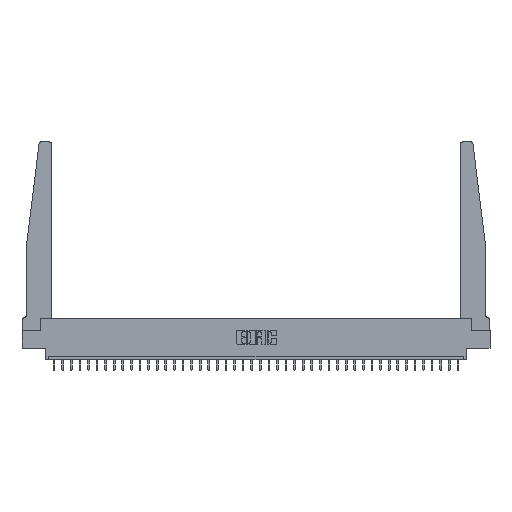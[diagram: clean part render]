
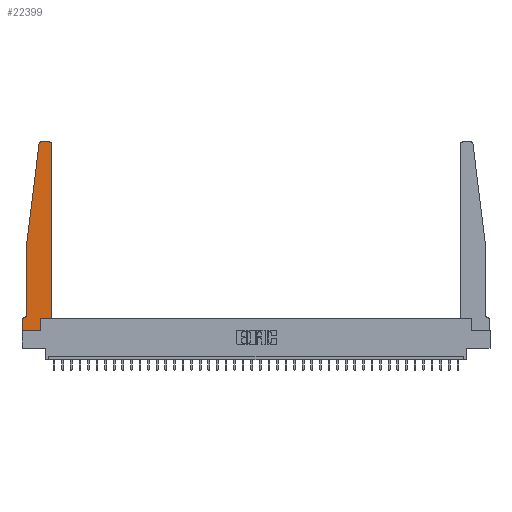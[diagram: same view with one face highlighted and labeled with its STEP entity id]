
A CAD part, top view. The second image highlights one B-rep face of the part: STEP entity #22399.
In plain terms, the highlighted planar face has unit normal (0, 0, 1).
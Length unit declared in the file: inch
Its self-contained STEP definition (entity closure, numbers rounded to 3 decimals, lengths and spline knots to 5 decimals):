
#115 = CARTESIAN_POINT ( 'NONE',  ( 0., 0.1875, 0.37 ) ) ;
#908 = EDGE_CURVE ( 'NONE', #25852, #27586, #5501, .T. ) ;
#1175 = ORIENTED_EDGE ( 'NONE', *, *, #10447, .T. ) ;
#1388 = CARTESIAN_POINT ( 'NONE',  ( 0.065, 0.2375, 0.37 ) ) ;
#1649 = ORIENTED_EDGE ( 'NONE', *, *, #10105, .T. ) ;
#2391 = DIRECTION ( 'NONE',  ( 1., 0., 0. ) ) ;
#2569 = EDGE_CURVE ( 'NONE', #26002, #22386, #15939, .T. ) ;
#2684 = EDGE_LOOP ( 'NONE', ( #1175, #7635, #31317, #21921, #1649, #19439, #5986, #26265, #10682, #6630, #33146, #14178 ) ) ;
#2781 = DIRECTION ( 'NONE',  ( -0.122, -0.992, 0. ) ) ;
#2871 = DIRECTION ( 'NONE',  ( 1., 0., 0. ) ) ;
#3240 = CARTESIAN_POINT ( 'NONE',  ( 0., 0., 0.37 ) ) ;
#3518 = DIRECTION ( 'NONE',  ( -1., 0., 0. ) ) ;
#3738 = VERTEX_POINT ( 'NONE', #9937 ) ;
#5237 = VERTEX_POINT ( 'NONE', #1388 ) ;
#5501 = LINE ( 'NONE', #33476, #26799 ) ;
#5986 = ORIENTED_EDGE ( 'NONE', *, *, #18563, .T. ) ;
#6097 = DIRECTION ( 'NONE',  ( 1., 0., 0. ) ) ;
#6144 = LINE ( 'NONE', #13271, #27427 ) ;
#6479 = LINE ( 'NONE', #33144, #17065 ) ;
#6630 = ORIENTED_EDGE ( 'NONE', *, *, #33755, .T. ) ;
#7582 = DIRECTION ( 'NONE',  ( 0., 1., 0. ) ) ;
#7635 = ORIENTED_EDGE ( 'NONE', *, *, #25223, .T. ) ;
#7638 = DIRECTION ( 'NONE',  ( 0., 0., 1. ) ) ;
#7783 = CARTESIAN_POINT ( 'NONE',  ( 0.27653, 2.72, 0.37 ) ) ;
#7954 = VECTOR ( 'NONE', #14132, 39.37008 ) ;
#8018 = VERTEX_POINT ( 'NONE', #28484 ) ;
#8507 = EDGE_CURVE ( 'NONE', #25192, #3738, #6144, .T. ) ;
#8789 = CARTESIAN_POINT ( 'NONE',  ( 0.065, 0.1875, 0.37 ) ) ;
#9550 = LINE ( 'NONE', #8789, #7954 ) ;
#9937 = CARTESIAN_POINT ( 'NONE',  ( 0.2605, 0.18, 0.37 ) ) ;
#10105 = EDGE_CURVE ( 'NONE', #5237, #8018, #24461, .T. ) ;
#10122 = CARTESIAN_POINT ( 'NONE',  ( 0.065, 1.25, 0.37 ) ) ;
#10183 = VECTOR ( 'NONE', #2391, 39.37008 ) ;
#10243 = DIRECTION ( 'NONE',  ( 1., 0., 0. ) ) ;
#10447 = EDGE_CURVE ( 'NONE', #22364, #23168, #29359, .T. ) ;
#10663 = VECTOR ( 'NONE', #2781, 39.37008 ) ;
#10682 = ORIENTED_EDGE ( 'NONE', *, *, #8507, .T. ) ;
#11725 = CIRCLE ( 'NONE', #15784, 0.03 ) ;
#12204 = LINE ( 'NONE', #16810, #29873 ) ;
#12744 = CARTESIAN_POINT ( 'NONE',  ( 0.015, 0.2375, 0.37 ) ) ;
#13271 = CARTESIAN_POINT ( 'NONE',  ( 0.2605, 0.18, 0.37 ) ) ;
#13623 = EDGE_CURVE ( 'NONE', #8018, #24699, #9550, .T. ) ;
#14040 = CARTESIAN_POINT ( 'NONE',  ( 0.27653, 2.75, 0.37 ) ) ;
#14132 = DIRECTION ( 'NONE',  ( -1., 0., 0. ) ) ;
#14178 = ORIENTED_EDGE ( 'NONE', *, *, #23310, .T. ) ;
#14276 = DIRECTION ( 'NONE',  ( 0., -1., 0. ) ) ;
#15290 = AXIS2_PLACEMENT_3D ( 'NONE', #12744, #20502, #15585 ) ;
#15353 = DIRECTION ( 'NONE',  ( 0., 0., 1. ) ) ;
#15585 = DIRECTION ( 'NONE',  ( -1., 0., 0. ) ) ;
#15628 = CARTESIAN_POINT ( 'NONE',  ( 0.065, 1.25, 0.37 ) ) ;
#15784 = AXIS2_PLACEMENT_3D ( 'NONE', #7783, #31130, #2871 ) ;
#15810 = CARTESIAN_POINT ( 'NONE',  ( 0.425, 0.18, 0.37 ) ) ;
#15939 = LINE ( 'NONE', #15628, #10663 ) ;
#16810 = CARTESIAN_POINT ( 'NONE',  ( 0.065, 1.25, 0.37 ) ) ;
#17065 = VECTOR ( 'NONE', #31494, 39.37008 ) ;
#18011 = CARTESIAN_POINT ( 'NONE',  ( 0.425, 0.18, 0.37 ) ) ;
#18563 = EDGE_CURVE ( 'NONE', #24699, #32704, #6479, .T. ) ;
#18902 = CARTESIAN_POINT ( 'NONE',  ( 0.24675, 2.72367, 0.37 ) ) ;
#19034 = CARTESIAN_POINT ( 'NONE',  ( 0.25, 2.75, 0.37 ) ) ;
#19439 = ORIENTED_EDGE ( 'NONE', *, *, #13623, .T. ) ;
#19564 = VECTOR ( 'NONE', #6097, 39.37008 ) ;
#19966 = CARTESIAN_POINT ( 'NONE',  ( 0.425, 2.72, 0.37 ) ) ;
#20502 = DIRECTION ( 'NONE',  ( 0., 0., -1. ) ) ;
#20621 = DIRECTION ( 'NONE',  ( 1., 0., 0. ) ) ;
#20883 = CARTESIAN_POINT ( 'NONE',  ( 0.2605, 0., 0.37 ) ) ;
#21921 = ORIENTED_EDGE ( 'NONE', *, *, #24023, .T. ) ;
#22006 = EDGE_CURVE ( 'NONE', #32704, #25192, #23709, .T. ) ;
#22024 = FACE_OUTER_BOUND ( 'NONE', #2684, .T. ) ;
#22364 = VERTEX_POINT ( 'NONE', #23070 ) ;
#22386 = VERTEX_POINT ( 'NONE', #10122 ) ;
#22399 = ADVANCED_FACE ( 'NONE', ( #22024 ), #25958, .T. ) ;
#23070 = CARTESIAN_POINT ( 'NONE',  ( 0.395, 2.75, 0.37 ) ) ;
#23168 = VERTEX_POINT ( 'NONE', #14040 ) ;
#23303 = CARTESIAN_POINT ( 'NONE',  ( 0.395, 2.72, 0.37 ) ) ;
#23310 = EDGE_CURVE ( 'NONE', #27586, #22364, #28707, .T. ) ;
#23709 = LINE ( 'NONE', #3240, #19564 ) ;
#24023 = EDGE_CURVE ( 'NONE', #22386, #5237, #12204, .T. ) ;
#24147 = LINE ( 'NONE', #18011, #10183 ) ;
#24461 = CIRCLE ( 'NONE', #15290, 0.05 ) ;
#24699 = VERTEX_POINT ( 'NONE', #115 ) ;
#25192 = VERTEX_POINT ( 'NONE', #20883 ) ;
#25223 = EDGE_CURVE ( 'NONE', #23168, #26002, #11725, .T. ) ;
#25852 = VERTEX_POINT ( 'NONE', #15810 ) ;
#25958 = PLANE ( 'NONE',  #28948 ) ;
#26002 = VERTEX_POINT ( 'NONE', #18902 ) ;
#26265 = ORIENTED_EDGE ( 'NONE', *, *, #22006, .T. ) ;
#26799 = VECTOR ( 'NONE', #7582, 39.37008 ) ;
#27427 = VECTOR ( 'NONE', #29116, 39.37008 ) ;
#27586 = VERTEX_POINT ( 'NONE', #19966 ) ;
#28484 = CARTESIAN_POINT ( 'NONE',  ( 0.015, 0.1875, 0.37 ) ) ;
#28707 = CIRCLE ( 'NONE', #29866, 0.03 ) ;
#28919 = VECTOR ( 'NONE', #3518, 39.37008 ) ;
#28948 = AXIS2_PLACEMENT_3D ( 'NONE', #31110, #15353, #20621 ) ;
#29116 = DIRECTION ( 'NONE',  ( 0., 1., 0. ) ) ;
#29359 = LINE ( 'NONE', #19034, #28919 ) ;
#29866 = AXIS2_PLACEMENT_3D ( 'NONE', #23303, #7638, #10243 ) ;
#29873 = VECTOR ( 'NONE', #14276, 39.37008 ) ;
#30974 = CARTESIAN_POINT ( 'NONE',  ( 0., 0., 0.37 ) ) ;
#31110 = CARTESIAN_POINT ( 'NONE',  ( 0., 0.1875, 0.37 ) ) ;
#31130 = DIRECTION ( 'NONE',  ( 0., 0., 1. ) ) ;
#31317 = ORIENTED_EDGE ( 'NONE', *, *, #2569, .T. ) ;
#31494 = DIRECTION ( 'NONE',  ( 0., -1., 0. ) ) ;
#32704 = VERTEX_POINT ( 'NONE', #30974 ) ;
#33144 = CARTESIAN_POINT ( 'NONE',  ( 0., 0., 0.37 ) ) ;
#33146 = ORIENTED_EDGE ( 'NONE', *, *, #908, .T. ) ;
#33476 = CARTESIAN_POINT ( 'NONE',  ( 0.425, 0.18, 0.37 ) ) ;
#33755 = EDGE_CURVE ( 'NONE', #3738, #25852, #24147, .T. ) ;
